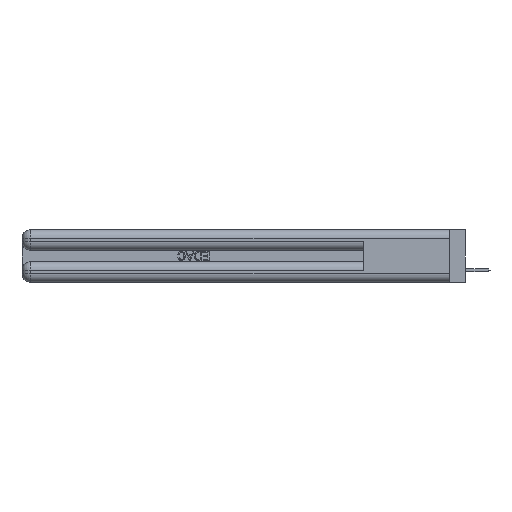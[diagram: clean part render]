
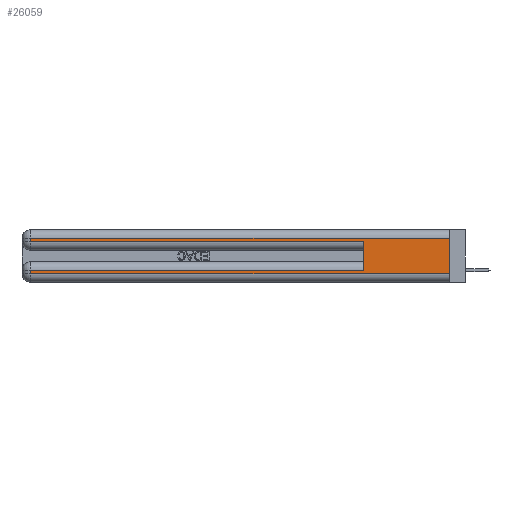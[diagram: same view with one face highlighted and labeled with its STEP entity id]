
A CAD part, left-side view. The second image highlights one B-rep face of the part: STEP entity #26059.
In plain terms, the highlighted planar face has unit normal (-1, 0, 0).
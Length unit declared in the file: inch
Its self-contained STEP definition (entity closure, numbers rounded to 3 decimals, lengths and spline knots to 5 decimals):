
#2159 = CARTESIAN_POINT ( 'NONE',  ( 0., 0., 0.085 ) ) ;
#2280 = EDGE_CURVE ( 'NONE', #42679, #40168, #13532, .T. ) ;
#2936 = LINE ( 'NONE', #31405, #23842 ) ;
#3412 = EDGE_CURVE ( 'NONE', #31796, #4521, #19426, .T. ) ;
#4377 = VECTOR ( 'NONE', #11810, 39.37008 ) ;
#4521 = VERTEX_POINT ( 'NONE', #19026 ) ;
#6814 = VECTOR ( 'NONE', #14503, 39.37008 ) ;
#6899 = EDGE_CURVE ( 'NONE', #21365, #40168, #2936, .T. ) ;
#6944 = LINE ( 'NONE', #40541, #36475 ) ;
#9853 = VECTOR ( 'NONE', #18283, 39.37008 ) ;
#9951 = ORIENTED_EDGE ( 'NONE', *, *, #3412, .T. ) ;
#10105 = EDGE_CURVE ( 'NONE', #35010, #40033, #6944, .T. ) ;
#10343 = CARTESIAN_POINT ( 'NONE',  ( 0., 2.94, 0.085 ) ) ;
#11285 = EDGE_CURVE ( 'NONE', #21365, #36887, #14315, .T. ) ;
#11810 = DIRECTION ( 'NONE',  ( 0., -1., 0. ) ) ;
#12404 = CARTESIAN_POINT ( 'NONE',  ( 0., 0.6, 0.085 ) ) ;
#12532 = LINE ( 'NONE', #18449, #9853 ) ;
#13532 = LINE ( 'NONE', #18292, #4377 ) ;
#14315 = LINE ( 'NONE', #2159, #30931 ) ;
#14503 = DIRECTION ( 'NONE',  ( 0., 0., -1. ) ) ;
#15483 = AXIS2_PLACEMENT_3D ( 'NONE', #37889, #20823, #41074 ) ;
#16786 = ORIENTED_EDGE ( 'NONE', *, *, #6899, .F. ) ;
#17063 = ORIENTED_EDGE ( 'NONE', *, *, #25098, .T. ) ;
#17998 = EDGE_CURVE ( 'NONE', #36887, #31796, #41697, .T. ) ;
#18283 = DIRECTION ( 'NONE',  ( 0., 0., -1. ) ) ;
#18292 = CARTESIAN_POINT ( 'NONE',  ( 0., 0., 0.285 ) ) ;
#18449 = CARTESIAN_POINT ( 'NONE',  ( 0., 0., 0.37 ) ) ;
#19026 = CARTESIAN_POINT ( 'NONE',  ( 0., 0., 0.06 ) ) ;
#19426 = LINE ( 'NONE', #27267, #37659 ) ;
#19612 = DIRECTION ( 'NONE',  ( 0., 1., 0. ) ) ;
#20823 = DIRECTION ( 'NONE',  ( 1., 0., 0. ) ) ;
#21030 = ORIENTED_EDGE ( 'NONE', *, *, #10105, .T. ) ;
#21365 = VERTEX_POINT ( 'NONE', #12404 ) ;
#23842 = VECTOR ( 'NONE', #24808, 39.37008 ) ;
#24808 = DIRECTION ( 'NONE',  ( 0., 0., 1. ) ) ;
#25098 = EDGE_CURVE ( 'NONE', #40033, #42679, #32849, .T. ) ;
#26059 = ADVANCED_FACE ( 'NONE', ( #38545 ), #37337, .F. ) ;
#27267 = CARTESIAN_POINT ( 'NONE',  ( 0., 0., 0.06 ) ) ;
#27522 = CARTESIAN_POINT ( 'NONE',  ( 0., 0.6, 0.285 ) ) ;
#29040 = EDGE_CURVE ( 'NONE', #35010, #4521, #12532, .T. ) ;
#29234 = DIRECTION ( 'NONE',  ( 0., 0., -1. ) ) ;
#29581 = ORIENTED_EDGE ( 'NONE', *, *, #2280, .T. ) ;
#30931 = VECTOR ( 'NONE', #19612, 39.37008 ) ;
#31405 = CARTESIAN_POINT ( 'NONE',  ( 0., 0.6, 0.145 ) ) ;
#31796 = VERTEX_POINT ( 'NONE', #32290 ) ;
#32290 = CARTESIAN_POINT ( 'NONE',  ( 0., 2.94, 0.06 ) ) ;
#32849 = LINE ( 'NONE', #42910, #43438 ) ;
#33523 = CARTESIAN_POINT ( 'NONE',  ( 0., 0., 0.31 ) ) ;
#35010 = VERTEX_POINT ( 'NONE', #33523 ) ;
#35051 = ORIENTED_EDGE ( 'NONE', *, *, #11285, .T. ) ;
#35129 = ORIENTED_EDGE ( 'NONE', *, *, #29040, .F. ) ;
#36475 = VECTOR ( 'NONE', #38082, 39.37008 ) ;
#36887 = VERTEX_POINT ( 'NONE', #10343 ) ;
#37337 = PLANE ( 'NONE',  #15483 ) ;
#37468 = CARTESIAN_POINT ( 'NONE',  ( 0., 2.94, 0.285 ) ) ;
#37501 = CARTESIAN_POINT ( 'NONE',  ( 0., 2.94, 0.31 ) ) ;
#37659 = VECTOR ( 'NONE', #40974, 39.37008 ) ;
#37889 = CARTESIAN_POINT ( 'NONE',  ( 0., 0., 0.37 ) ) ;
#38082 = DIRECTION ( 'NONE',  ( 0., 1., 0. ) ) ;
#38357 = CARTESIAN_POINT ( 'NONE',  ( 0., 2.94, 0.37 ) ) ;
#38545 = FACE_OUTER_BOUND ( 'NONE', #43271, .T. ) ;
#40033 = VERTEX_POINT ( 'NONE', #37501 ) ;
#40168 = VERTEX_POINT ( 'NONE', #27522 ) ;
#40541 = CARTESIAN_POINT ( 'NONE',  ( 0., 0., 0.31 ) ) ;
#40974 = DIRECTION ( 'NONE',  ( 0., -1., 0. ) ) ;
#41074 = DIRECTION ( 'NONE',  ( 0., 0., -1. ) ) ;
#41697 = LINE ( 'NONE', #38357, #6814 ) ;
#42507 = ORIENTED_EDGE ( 'NONE', *, *, #17998, .T. ) ;
#42679 = VERTEX_POINT ( 'NONE', #37468 ) ;
#42910 = CARTESIAN_POINT ( 'NONE',  ( 0., 2.94, 0.37 ) ) ;
#43271 = EDGE_LOOP ( 'NONE', ( #35129, #21030, #17063, #29581, #16786, #35051, #42507, #9951 ) ) ;
#43438 = VECTOR ( 'NONE', #29234, 39.37008 ) ;
